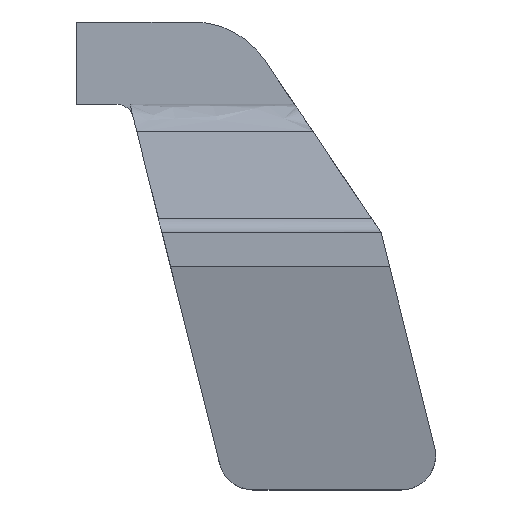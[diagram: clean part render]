
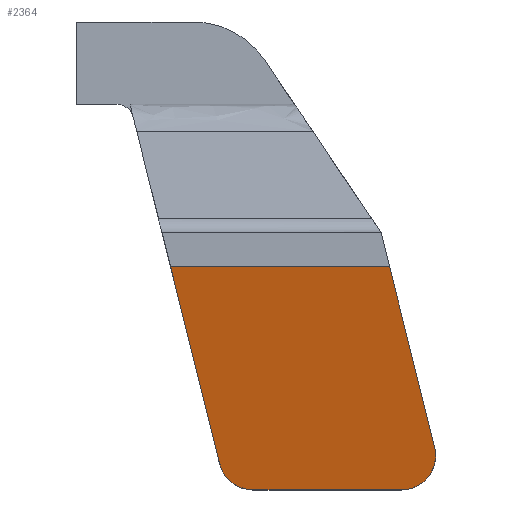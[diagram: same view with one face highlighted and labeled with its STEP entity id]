
A CAD part, top view. The second image highlights one B-rep face of the part: STEP entity #2364.
In plain terms, the highlighted planar face has unit normal (0, -0.218, 0.976).
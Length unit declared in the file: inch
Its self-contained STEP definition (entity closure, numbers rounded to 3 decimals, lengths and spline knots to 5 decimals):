
#20 = CARTESIAN_POINT ( 'NONE',  ( -4.19534, -0.72057, 0.15656 ) ) ;
#54 = CARTESIAN_POINT ( 'NONE',  ( -3.57702, -0.65, 0.17231 ) ) ;
#64 = VERTEX_POINT ( 'NONE', #1312 ) ;
#88 = EDGE_CURVE ( 'NONE', #2569, #217, #1673, .T. ) ;
#96 = ORIENTED_EDGE ( 'NONE', *, *, #88, .T. ) ;
#102 = PLANE ( 'NONE',  #1690 ) ;
#116 = CARTESIAN_POINT ( 'NONE',  ( -3.57702, -0.70858, 0.15924 ) ) ;
#169 = ORIENTED_EDGE ( 'NONE', *, *, #964, .T. ) ;
#217 = VERTEX_POINT ( 'NONE', #2997 ) ;
#266 = VECTOR ( 'NONE', #3379, 39.37008 ) ;
#311 = ORIENTED_EDGE ( 'NONE', *, *, #2832, .T. ) ;
#341 = CARTESIAN_POINT ( 'NONE',  ( -3.61844, -0.75, 0.15 ) ) ;
#812 = ORIENTED_EDGE ( 'NONE', *, *, #2087, .F. ) ;
#915 = VECTOR ( 'NONE', #3207, 39.37008 ) ;
#964 = EDGE_CURVE ( 'NONE', #1275, #3213, #1596, .T. ) ;
#1017 = LINE ( 'NONE', #2603, #266 ) ;
#1046 = CARTESIAN_POINT ( 'NONE',  ( -4.35007, -0.1, 0.295 ) ) ;
#1052 = CARTESIAN_POINT ( 'NONE',  ( -3.67702, -0.75, 0.15 ) ) ;
#1053 = CARTESIAN_POINT ( 'NONE',  ( -3.57801, -0.63373, 0.17594 ) ) ;
#1082 = CARTESIAN_POINT ( 'NONE',  ( -4.15767, -0.75, 0.15 ) ) ;
#1132 = DIRECTION ( 'NONE',  ( 1., 0., 0. ) ) ;
#1160 = CARTESIAN_POINT ( 'NONE',  ( -4.10988, -0.75, 0.15 ) ) ;
#1240 = ORIENTED_EDGE ( 'NONE', *, *, #2494, .T. ) ;
#1244 =( BOUNDED_CURVE ( )  B_SPLINE_CURVE ( 3, ( #1834, #3215, #1053, #1907 ),
 .UNSPECIFIED., .F., .T. ) 
 B_SPLINE_CURVE_WITH_KNOTS ( ( 4, 4 ),
 ( 4.71239, 4.95674 ),
 .UNSPECIFIED. ) 
 CURVE ( )  GEOMETRIC_REPRESENTATION_ITEM ( )  RATIONAL_B_SPLINE_CURVE ( ( 1., 0.995, 0.995, 1. ) ) 
 REPRESENTATION_ITEM ( '' )  );
#1275 = VERTEX_POINT ( 'NONE', #1052 ) ;
#1283 = CARTESIAN_POINT ( 'NONE',  ( -4.625, -0.75, 0.15 ) ) ;
#1312 = CARTESIAN_POINT ( 'NONE',  ( -4.20691, -0.67419, 0.16691 ) ) ;
#1451 = VERTEX_POINT ( 'NONE', #1160 ) ;
#1481 = LINE ( 'NONE', #1932, #3342 ) ;
#1521 = EDGE_LOOP ( 'NONE', ( #2334, #169, #1807, #96, #812, #1240, #311 ) ) ;
#1526 = LINE ( 'NONE', #1283, #1531 ) ;
#1531 = VECTOR ( 'NONE', #3272, 39.37008 ) ;
#1596 =( BOUNDED_CURVE ( )  B_SPLINE_CURVE ( 3, ( #1662, #341, #116, #1942 ),
 .UNSPECIFIED., .F., .T. ) 
 B_SPLINE_CURVE_WITH_KNOTS ( ( 4, 4 ),
 ( 3.14159, 4.71239 ),
 .UNSPECIFIED. ) 
 CURVE ( )  GEOMETRIC_REPRESENTATION_ITEM ( )  RATIONAL_B_SPLINE_CURVE ( ( 1., 0.805, 0.805, 1. ) ) 
 REPRESENTATION_ITEM ( '' )  );
#1637 = CARTESIAN_POINT ( 'NONE',  ( -3.71515, -0.08372, 0.29863 ) ) ;
#1648 = DIRECTION ( 'NONE',  ( 0., 0.976, 0.218 ) ) ;
#1662 = CARTESIAN_POINT ( 'NONE',  ( -3.67702, -0.75, 0.15 ) ) ;
#1673 = LINE ( 'NONE', #1637, #915 ) ;
#1690 = AXIS2_PLACEMENT_3D ( 'NONE', #3047, #2503, #1648 ) ;
#1807 = ORIENTED_EDGE ( 'NONE', *, *, #2258, .T. ) ;
#1834 = CARTESIAN_POINT ( 'NONE',  ( -3.57702, -0.65, 0.17231 ) ) ;
#1907 = CARTESIAN_POINT ( 'NONE',  ( -3.57999, -0.62581, 0.1777 ) ) ;
#1932 = CARTESIAN_POINT ( 'NONE',  ( -4.28377, -0.1, 0.295 ) ) ;
#1942 = CARTESIAN_POINT ( 'NONE',  ( -3.57702, -0.65, 0.17231 ) ) ;
#1997 = FACE_OUTER_BOUND ( 'NONE', #1521, .T. ) ;
#2071 = CARTESIAN_POINT ( 'NONE',  ( -4.20691, -0.67419, 0.16691 ) ) ;
#2087 = EDGE_CURVE ( 'NONE', #2836, #217, #1481, .T. ) ;
#2258 = EDGE_CURVE ( 'NONE', #3213, #2569, #1244, .T. ) ;
#2334 = ORIENTED_EDGE ( 'NONE', *, *, #3325, .T. ) ;
#2364 = ADVANCED_FACE ( 'NONE', ( #1997 ), #102, .F. ) ;
#2494 = EDGE_CURVE ( 'NONE', #2836, #64, #1017, .T. ) ;
#2503 = DIRECTION ( 'NONE',  ( 0., 0.218, -0.976 ) ) ;
#2541 =( BOUNDED_CURVE ( )  B_SPLINE_CURVE ( 3, ( #2071, #20, #1082, #3123 ),
 .UNSPECIFIED., .F., .F. ) 
 B_SPLINE_CURVE_WITH_KNOTS ( ( 4, 4 ),
 ( 1.81514, 3.14159 ),
 .UNSPECIFIED. ) 
 CURVE ( )  GEOMETRIC_REPRESENTATION_ITEM ( )  RATIONAL_B_SPLINE_CURVE ( ( 1., 0.859, 0.859, 1. ) ) 
 REPRESENTATION_ITEM ( '' )  );
#2569 = VERTEX_POINT ( 'NONE', #3275 ) ;
#2603 = CARTESIAN_POINT ( 'NONE',  ( -4.44344, 0.2745, 0.37854 ) ) ;
#2832 = EDGE_CURVE ( 'NONE', #64, #1451, #2541, .T. ) ;
#2836 = VERTEX_POINT ( 'NONE', #1046 ) ;
#2997 = CARTESIAN_POINT ( 'NONE',  ( -3.71109, -0.1, 0.295 ) ) ;
#3047 = CARTESIAN_POINT ( 'NONE',  ( -4.625, -0.1, 0.295 ) ) ;
#3123 = CARTESIAN_POINT ( 'NONE',  ( -4.10988, -0.75, 0.15 ) ) ;
#3207 = DIRECTION ( 'NONE',  ( -0.236, 0.948, 0.212 ) ) ;
#3213 = VERTEX_POINT ( 'NONE', #54 ) ;
#3215 = CARTESIAN_POINT ( 'NONE',  ( -3.57702, -0.64183, 0.17413 ) ) ;
#3272 = DIRECTION ( 'NONE',  ( 1., 0., 0. ) ) ;
#3275 = CARTESIAN_POINT ( 'NONE',  ( -3.57999, -0.62581, 0.1777 ) ) ;
#3325 = EDGE_CURVE ( 'NONE', #1451, #1275, #1526, .T. ) ;
#3342 = VECTOR ( 'NONE', #1132, 39.37008 ) ;
#3379 = DIRECTION ( 'NONE',  ( 0.236, -0.948, -0.212 ) ) ;
